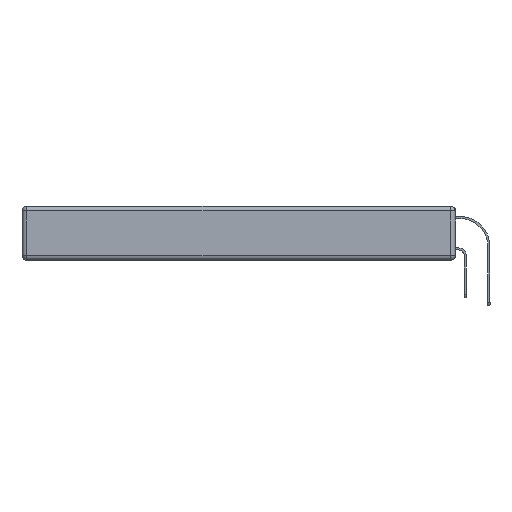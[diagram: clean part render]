
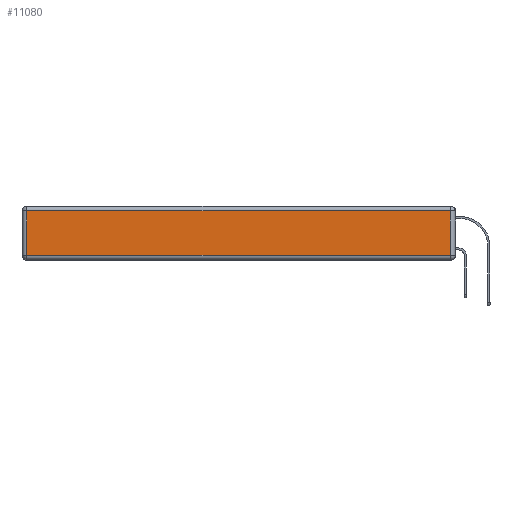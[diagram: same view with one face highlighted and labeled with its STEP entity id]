
A CAD part, left-side view. The second image highlights one B-rep face of the part: STEP entity #11080.
In plain terms, the highlighted planar face has unit normal (-1, 0, 0).
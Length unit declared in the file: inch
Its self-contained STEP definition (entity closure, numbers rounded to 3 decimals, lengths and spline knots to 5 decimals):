
#422 = CARTESIAN_POINT ( 'NONE',  ( 0., 2.75, -0.03 ) ) ;
#650 = DIRECTION ( 'NONE',  ( -1., 0., 0. ) ) ;
#665 = ORIENTED_EDGE ( 'NONE', *, *, #16081, .T. ) ;
#843 = VERTEX_POINT ( 'NONE', #17293 ) ;
#1403 = VERTEX_POINT ( 'NONE', #9048 ) ;
#1445 = ORIENTED_EDGE ( 'NONE', *, *, #7597, .T. ) ;
#1590 = DIRECTION ( 'NONE',  ( 0., 1., 0. ) ) ;
#1983 = CARTESIAN_POINT ( 'NONE',  ( 0., 0., -0.313 ) ) ;
#3436 = VECTOR ( 'NONE', #11952, 39.37008 ) ;
#3637 = CARTESIAN_POINT ( 'NONE',  ( 0., 0.03, -0.343 ) ) ;
#4908 = VECTOR ( 'NONE', #10782, 39.37008 ) ;
#5664 = VERTEX_POINT ( 'NONE', #16654 ) ;
#6246 = EDGE_CURVE ( 'NONE', #14176, #843, #12705, .T. ) ;
#6348 = ORIENTED_EDGE ( 'NONE', *, *, #6246, .T. ) ;
#6426 = LINE ( 'NONE', #3637, #3436 ) ;
#7597 = EDGE_CURVE ( 'NONE', #1403, #5664, #15967, .T. ) ;
#7605 = PLANE ( 'NONE',  #15706 ) ;
#7634 = ORIENTED_EDGE ( 'NONE', *, *, #14745, .T. ) ;
#8671 = VECTOR ( 'NONE', #1590, 39.37008 ) ;
#8984 = CARTESIAN_POINT ( 'NONE',  ( 0., 0.03, -0.03 ) ) ;
#9048 = CARTESIAN_POINT ( 'NONE',  ( 0., 2.72, -0.313 ) ) ;
#9787 = EDGE_LOOP ( 'NONE', ( #1445, #7634, #6348, #665 ) ) ;
#10782 = DIRECTION ( 'NONE',  ( 0., 0., -1. ) ) ;
#11080 = ADVANCED_FACE ( 'NONE', ( #14969 ), #7605, .T. ) ;
#11669 = CARTESIAN_POINT ( 'NONE',  ( 0., 0., -0.343 ) ) ;
#11952 = DIRECTION ( 'NONE',  ( 0., 0., 1. ) ) ;
#12287 = VECTOR ( 'NONE', #15785, 39.37008 ) ;
#12705 = LINE ( 'NONE', #422, #8671 ) ;
#13122 = DIRECTION ( 'NONE',  ( 0., 0., 1. ) ) ;
#14176 = VERTEX_POINT ( 'NONE', #8984 ) ;
#14745 = EDGE_CURVE ( 'NONE', #5664, #14176, #6426, .T. ) ;
#14969 = FACE_OUTER_BOUND ( 'NONE', #9787, .T. ) ;
#15706 = AXIS2_PLACEMENT_3D ( 'NONE', #11669, #650, #13122 ) ;
#15785 = DIRECTION ( 'NONE',  ( 0., -1., 0. ) ) ;
#15967 = LINE ( 'NONE', #1983, #12287 ) ;
#16081 = EDGE_CURVE ( 'NONE', #843, #1403, #16365, .T. ) ;
#16365 = LINE ( 'NONE', #17548, #4908 ) ;
#16654 = CARTESIAN_POINT ( 'NONE',  ( 0., 0.03, -0.313 ) ) ;
#17293 = CARTESIAN_POINT ( 'NONE',  ( 0., 2.72, -0.03 ) ) ;
#17548 = CARTESIAN_POINT ( 'NONE',  ( 0., 2.72, -0.343 ) ) ;
